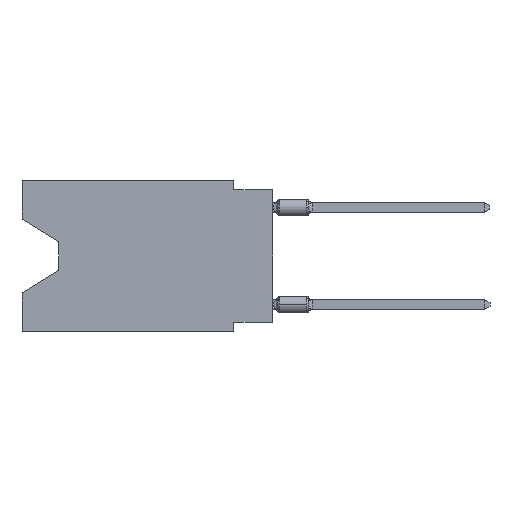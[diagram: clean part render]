
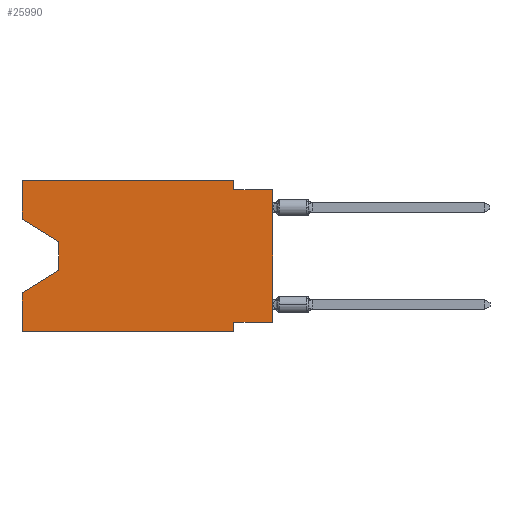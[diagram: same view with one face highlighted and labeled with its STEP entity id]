
A CAD part, left-side view. The second image highlights one B-rep face of the part: STEP entity #25990.
In plain terms, the highlighted planar face has unit normal (-1, 0, 0).
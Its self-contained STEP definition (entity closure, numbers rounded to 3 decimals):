
#16 = VERTEX_POINT ( 'NONE', #19428 ) ;
#74 = CARTESIAN_POINT ( 'NONE',  ( 0., 16.383, -9.906 ) ) ;
#565 = VERTEX_POINT ( 'NONE', #4349 ) ;
#1074 = DIRECTION ( 'NONE',  ( 0., 0., 1. ) ) ;
#1434 = LINE ( 'NONE', #19866, #2663 ) ;
#1747 = FACE_OUTER_BOUND ( 'NONE', #24285, .T. ) ;
#2096 = ORIENTED_EDGE ( 'NONE', *, *, #10451, .F. ) ;
#2437 = ORIENTED_EDGE ( 'NONE', *, *, #24694, .F. ) ;
#2544 = VECTOR ( 'NONE', #14543, 1000. ) ;
#2663 = VECTOR ( 'NONE', #18079, 1000. ) ;
#2666 = EDGE_CURVE ( 'NONE', #16, #9218, #25592, .T. ) ;
#3233 = VERTEX_POINT ( 'NONE', #9717 ) ;
#3823 = CARTESIAN_POINT ( 'NONE',  ( 0., 16.383, -2.546 ) ) ;
#3980 = CARTESIAN_POINT ( 'NONE',  ( 0., 2.54, 0. ) ) ;
#4233 = VECTOR ( 'NONE', #1074, 1000. ) ;
#4344 = EDGE_CURVE ( 'NONE', #12449, #10494, #8952, .T. ) ;
#4349 = CARTESIAN_POINT ( 'NONE',  ( 0., 2.54, -9.271 ) ) ;
#4577 = ORIENTED_EDGE ( 'NONE', *, *, #5692, .T. ) ;
#4635 = VECTOR ( 'NONE', #24375, 1000. ) ;
#4982 = DIRECTION ( 'NONE',  ( 0., 0., -1. ) ) ;
#5265 = EDGE_CURVE ( 'NONE', #565, #23402, #20579, .T. ) ;
#5569 = CARTESIAN_POINT ( 'NONE',  ( 0., 16.383, -9.906 ) ) ;
#5692 = EDGE_CURVE ( 'NONE', #24312, #3233, #1434, .T. ) ;
#6232 = ORIENTED_EDGE ( 'NONE', *, *, #25972, .F. ) ;
#7736 = CARTESIAN_POINT ( 'NONE',  ( 0., 16.383, 0. ) ) ;
#7752 = LINE ( 'NONE', #9538, #4233 ) ;
#7824 = DIRECTION ( 'NONE',  ( 0., -1., 0. ) ) ;
#8062 = ORIENTED_EDGE ( 'NONE', *, *, #2666, .T. ) ;
#8232 = EDGE_CURVE ( 'NONE', #25889, #23402, #16467, .T. ) ;
#8952 = LINE ( 'NONE', #15350, #22647 ) ;
#9218 = VERTEX_POINT ( 'NONE', #23792 ) ;
#9538 = CARTESIAN_POINT ( 'NONE',  ( 0., 16.383, 0. ) ) ;
#9703 = ORIENTED_EDGE ( 'NONE', *, *, #5265, .F. ) ;
#9717 = CARTESIAN_POINT ( 'NONE',  ( 0., 16.383, -7.36 ) ) ;
#10041 = VECTOR ( 'NONE', #26972, 1000. ) ;
#10451 = EDGE_CURVE ( 'NONE', #25889, #3233, #14145, .T. ) ;
#10474 = CARTESIAN_POINT ( 'NONE',  ( 0., 16.383, 0. ) ) ;
#10494 = VERTEX_POINT ( 'NONE', #11831 ) ;
#11107 = DIRECTION ( 'NONE',  ( 0., 0., 1. ) ) ;
#11634 = DIRECTION ( 'NONE',  ( 0., 0., -1. ) ) ;
#11831 = CARTESIAN_POINT ( 'NONE',  ( 0., 2.54, -0.635 ) ) ;
#12449 = VERTEX_POINT ( 'NONE', #3980 ) ;
#13300 = CARTESIAN_POINT ( 'NONE',  ( 0., 16.383, 0. ) ) ;
#13846 = ORIENTED_EDGE ( 'NONE', *, *, #25017, .F. ) ;
#14056 = LINE ( 'NONE', #3823, #24756 ) ;
#14145 = LINE ( 'NONE', #7736, #10041 ) ;
#14214 = VERTEX_POINT ( 'NONE', #19158 ) ;
#14237 = VECTOR ( 'NONE', #7824, 1000. ) ;
#14312 = DIRECTION ( 'NONE',  ( 0., -0.855, -0.519 ) ) ;
#14543 = DIRECTION ( 'NONE',  ( 0., -1., 0. ) ) ;
#14555 = DIRECTION ( 'NONE',  ( 1., 0., 0. ) ) ;
#15350 = CARTESIAN_POINT ( 'NONE',  ( 0., 2.54, 0. ) ) ;
#15549 = LINE ( 'NONE', #21714, #24463 ) ;
#16165 = ORIENTED_EDGE ( 'NONE', *, *, #21765, .F. ) ;
#16467 = LINE ( 'NONE', #74, #2544 ) ;
#17265 = VERTEX_POINT ( 'NONE', #13300 ) ;
#17388 = CARTESIAN_POINT ( 'NONE',  ( 0., 0., 0. ) ) ;
#17914 = LINE ( 'NONE', #24203, #25803 ) ;
#18079 = DIRECTION ( 'NONE',  ( 0., 0.855, -0.519 ) ) ;
#18085 = LINE ( 'NONE', #26415, #4635 ) ;
#18254 = VERTEX_POINT ( 'NONE', #18269 ) ;
#18269 = CARTESIAN_POINT ( 'NONE',  ( 0., 16.383, -2.546 ) ) ;
#18287 = ORIENTED_EDGE ( 'NONE', *, *, #22611, .T. ) ;
#19158 = CARTESIAN_POINT ( 'NONE',  ( 0., 13.97, -4.013 ) ) ;
#19385 = VECTOR ( 'NONE', #11107, 1000. ) ;
#19428 = CARTESIAN_POINT ( 'NONE',  ( 0., 0., -9.271 ) ) ;
#19866 = CARTESIAN_POINT ( 'NONE',  ( 0., 13.97, -5.893 ) ) ;
#20574 = ORIENTED_EDGE ( 'NONE', *, *, #8232, .T. ) ;
#20579 = LINE ( 'NONE', #22620, #22265 ) ;
#21714 = CARTESIAN_POINT ( 'NONE',  ( 0., 0., -9.271 ) ) ;
#21765 = EDGE_CURVE ( 'NONE', #16, #565, #15549, .T. ) ;
#22032 = CARTESIAN_POINT ( 'NONE',  ( 0., 0., -0.635 ) ) ;
#22054 = ORIENTED_EDGE ( 'NONE', *, *, #4344, .F. ) ;
#22087 = DIRECTION ( 'NONE',  ( 0., 0., -1. ) ) ;
#22265 = VECTOR ( 'NONE', #22087, 1000. ) ;
#22531 = CARTESIAN_POINT ( 'NONE',  ( 0., 13.97, -5.893 ) ) ;
#22611 = EDGE_CURVE ( 'NONE', #14214, #24312, #17914, .T. ) ;
#22620 = CARTESIAN_POINT ( 'NONE',  ( 0., 2.54, -9.906 ) ) ;
#22632 = PLANE ( 'NONE',  #22982 ) ;
#22647 = VECTOR ( 'NONE', #4982, 1000. ) ;
#22982 = AXIS2_PLACEMENT_3D ( 'NONE', #10474, #14555, #26859 ) ;
#23212 = EDGE_CURVE ( 'NONE', #18254, #14214, #14056, .T. ) ;
#23326 = CARTESIAN_POINT ( 'NONE',  ( 0., 2.54, -9.906 ) ) ;
#23402 = VERTEX_POINT ( 'NONE', #23326 ) ;
#23761 = DIRECTION ( 'NONE',  ( 0., 1., 0. ) ) ;
#23792 = CARTESIAN_POINT ( 'NONE',  ( 0., 0., -0.635 ) ) ;
#24203 = CARTESIAN_POINT ( 'NONE',  ( 0., 13.97, -4.013 ) ) ;
#24285 = EDGE_LOOP ( 'NONE', ( #25191, #18287, #4577, #2096, #20574, #9703, #16165, #8062, #13846, #22054, #2437, #6232 ) ) ;
#24312 = VERTEX_POINT ( 'NONE', #22531 ) ;
#24375 = DIRECTION ( 'NONE',  ( 0., -1., 0. ) ) ;
#24463 = VECTOR ( 'NONE', #23761, 1000. ) ;
#24694 = EDGE_CURVE ( 'NONE', #17265, #12449, #18085, .T. ) ;
#24756 = VECTOR ( 'NONE', #14312, 1000. ) ;
#25017 = EDGE_CURVE ( 'NONE', #10494, #9218, #26253, .T. ) ;
#25191 = ORIENTED_EDGE ( 'NONE', *, *, #23212, .T. ) ;
#25592 = LINE ( 'NONE', #17388, #19385 ) ;
#25803 = VECTOR ( 'NONE', #11634, 1000. ) ;
#25889 = VERTEX_POINT ( 'NONE', #5569 ) ;
#25972 = EDGE_CURVE ( 'NONE', #18254, #17265, #7752, .T. ) ;
#25990 = ADVANCED_FACE ( 'NONE', ( #1747 ), #22632, .F. ) ;
#26253 = LINE ( 'NONE', #22032, #14237 ) ;
#26415 = CARTESIAN_POINT ( 'NONE',  ( 0., 16.383, 0. ) ) ;
#26859 = DIRECTION ( 'NONE',  ( 0., 0., -1. ) ) ;
#26972 = DIRECTION ( 'NONE',  ( 0., 0., 1. ) ) ;
